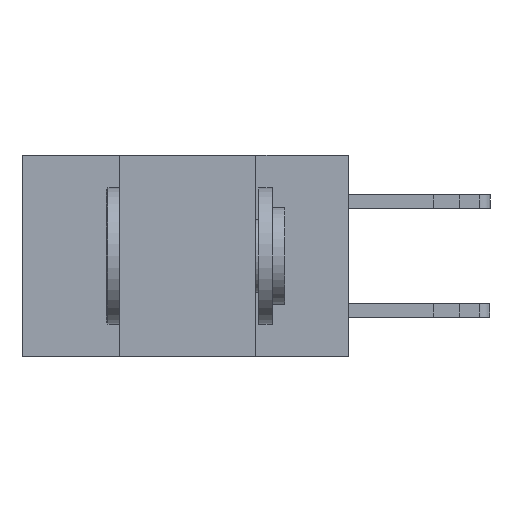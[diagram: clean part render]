
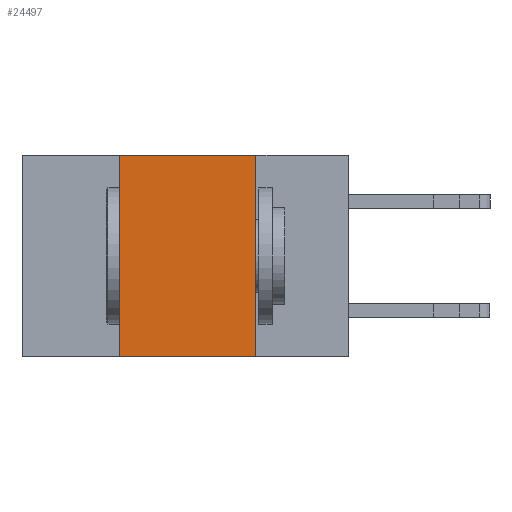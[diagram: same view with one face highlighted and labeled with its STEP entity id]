
A CAD part, left-side view. The second image highlights one B-rep face of the part: STEP entity #24497.
In plain terms, the highlighted planar face has unit normal (-1, 0, 0).
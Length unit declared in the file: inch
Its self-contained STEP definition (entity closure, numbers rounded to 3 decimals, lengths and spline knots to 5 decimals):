
#623 = DIRECTION ( 'NONE',  ( 0., 0., -1. ) ) ;
#1417 = VECTOR ( 'NONE', #623, 39.37008 ) ;
#2072 = LINE ( 'NONE', #26271, #24007 ) ;
#3171 = CARTESIAN_POINT ( 'NONE',  ( 0., 0.42, -0.37 ) ) ;
#6069 = CARTESIAN_POINT ( 'NONE',  ( 0., 0.42, 0. ) ) ;
#6847 = EDGE_CURVE ( 'NONE', #21288, #9112, #2072, .T. ) ;
#7223 = VERTEX_POINT ( 'NONE', #16472 ) ;
#7835 = VECTOR ( 'NONE', #14256, 39.37008 ) ;
#8641 = DIRECTION ( 'NONE',  ( 0., -1., 0. ) ) ;
#8856 = EDGE_LOOP ( 'NONE', ( #14016, #15416, #26015, #22982 ) ) ;
#8959 = EDGE_CURVE ( 'NONE', #20854, #7223, #20364, .T. ) ;
#9091 = CARTESIAN_POINT ( 'NONE',  ( 0., 0.17, 0. ) ) ;
#9112 = VERTEX_POINT ( 'NONE', #22917 ) ;
#9698 = DIRECTION ( 'NONE',  ( 1., 0., 0. ) ) ;
#9709 = CARTESIAN_POINT ( 'NONE',  ( 0., 0.6, 0. ) ) ;
#11388 = AXIS2_PLACEMENT_3D ( 'NONE', #16073, #9698, #24578 ) ;
#12581 = EDGE_CURVE ( 'NONE', #21288, #20854, #13507, .T. ) ;
#13507 = LINE ( 'NONE', #14159, #7835 ) ;
#14016 = ORIENTED_EDGE ( 'NONE', *, *, #26778, .F. ) ;
#14159 = CARTESIAN_POINT ( 'NONE',  ( 0., 0.42, 0. ) ) ;
#14256 = DIRECTION ( 'NONE',  ( 0., 0., 1. ) ) ;
#15416 = ORIENTED_EDGE ( 'NONE', *, *, #8959, .F. ) ;
#16073 = CARTESIAN_POINT ( 'NONE',  ( 0., 0.6, 0. ) ) ;
#16472 = CARTESIAN_POINT ( 'NONE',  ( 0., 0.17, 0. ) ) ;
#17905 = FACE_OUTER_BOUND ( 'NONE', #8856, .T. ) ;
#20364 = LINE ( 'NONE', #9709, #25970 ) ;
#20740 = LINE ( 'NONE', #9091, #1417 ) ;
#20854 = VERTEX_POINT ( 'NONE', #6069 ) ;
#21288 = VERTEX_POINT ( 'NONE', #3171 ) ;
#22454 = PLANE ( 'NONE',  #11388 ) ;
#22464 = DIRECTION ( 'NONE',  ( 0., -1., 0. ) ) ;
#22917 = CARTESIAN_POINT ( 'NONE',  ( 0., 0.17, -0.37 ) ) ;
#22982 = ORIENTED_EDGE ( 'NONE', *, *, #6847, .T. ) ;
#24007 = VECTOR ( 'NONE', #8641, 39.37008 ) ;
#24497 = ADVANCED_FACE ( 'NONE', ( #17905 ), #22454, .F. ) ;
#24578 = DIRECTION ( 'NONE',  ( 0., 0., -1. ) ) ;
#25970 = VECTOR ( 'NONE', #22464, 39.37008 ) ;
#26015 = ORIENTED_EDGE ( 'NONE', *, *, #12581, .F. ) ;
#26271 = CARTESIAN_POINT ( 'NONE',  ( 0., 0.6, -0.37 ) ) ;
#26778 = EDGE_CURVE ( 'NONE', #7223, #9112, #20740, .T. ) ;
